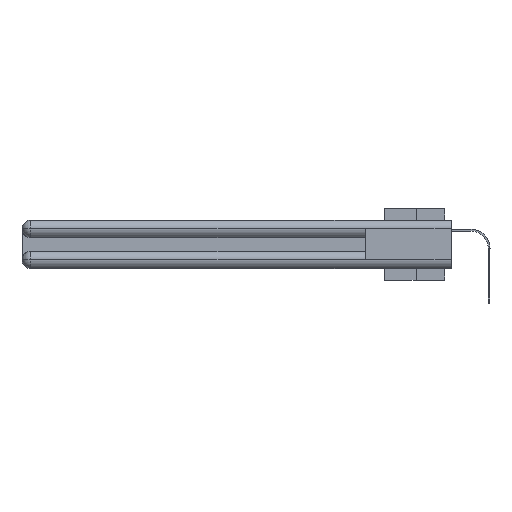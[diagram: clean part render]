
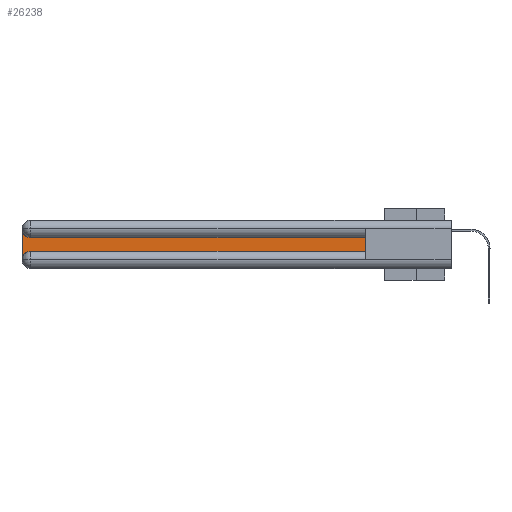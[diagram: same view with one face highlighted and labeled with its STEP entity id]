
A CAD part, left-side view. The second image highlights one B-rep face of the part: STEP entity #26238.
In plain terms, the highlighted planar face has unit normal (-1, 0, 0).
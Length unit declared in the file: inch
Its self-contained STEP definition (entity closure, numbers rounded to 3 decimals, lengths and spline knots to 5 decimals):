
#18 = CARTESIAN_POINT ( 'NONE',  ( 0.075, 2.94, -0.2775 ) ) ;
#342 = CIRCLE ( 'NONE', #5447, 0.06 ) ;
#403 = ORIENTED_EDGE ( 'NONE', *, *, #12688, .T. ) ;
#964 = CARTESIAN_POINT ( 'NONE',  ( 0.075, 0.6, -0.2175 ) ) ;
#1735 = LINE ( 'NONE', #29291, #29324 ) ;
#1938 = VERTEX_POINT ( 'NONE', #13409 ) ;
#2490 = VERTEX_POINT ( 'NONE', #15126 ) ;
#3595 = VERTEX_POINT ( 'NONE', #4472 ) ;
#3996 = DIRECTION ( 'NONE',  ( 0., -1., 0. ) ) ;
#4472 = CARTESIAN_POINT ( 'NONE',  ( 0.075, 3., -0.2775 ) ) ;
#5447 = AXIS2_PLACEMENT_3D ( 'NONE', #18, #12202, #24396 ) ;
#5637 = ORIENTED_EDGE ( 'NONE', *, *, #17181, .T. ) ;
#7115 = EDGE_CURVE ( 'NONE', #2490, #18605, #31381, .T. ) ;
#8290 = VERTEX_POINT ( 'NONE', #36392 ) ;
#10397 = CARTESIAN_POINT ( 'NONE',  ( 0.075, 0.6, -0.1225 ) ) ;
#10613 = DIRECTION ( 'NONE',  ( 0., 1., 0. ) ) ;
#11081 = EDGE_LOOP ( 'NONE', ( #22307, #5637, #36394, #403, #11160, #30911 ) ) ;
#11160 = ORIENTED_EDGE ( 'NONE', *, *, #7115, .T. ) ;
#12202 = DIRECTION ( 'NONE',  ( 1., 0., 0. ) ) ;
#12688 = EDGE_CURVE ( 'NONE', #3595, #2490, #342, .T. ) ;
#13157 = DIRECTION ( 'NONE',  ( 0., 0., -1. ) ) ;
#13409 = CARTESIAN_POINT ( 'NONE',  ( 0.075, 2.94, -0.1225 ) ) ;
#13956 = EDGE_CURVE ( 'NONE', #14171, #1938, #31977, .T. ) ;
#14117 = FACE_OUTER_BOUND ( 'NONE', #11081, .T. ) ;
#14171 = VERTEX_POINT ( 'NONE', #35559 ) ;
#15126 = CARTESIAN_POINT ( 'NONE',  ( 0.075, 2.94, -0.2175 ) ) ;
#15344 = AXIS2_PLACEMENT_3D ( 'NONE', #32674, #19718, #37900 ) ;
#15754 = VECTOR ( 'NONE', #10613, 39.37008 ) ;
#17181 = EDGE_CURVE ( 'NONE', #1938, #8290, #27856, .T. ) ;
#18309 = EDGE_CURVE ( 'NONE', #18605, #14171, #26946, .T. ) ;
#18605 = VERTEX_POINT ( 'NONE', #964 ) ;
#19331 = CARTESIAN_POINT ( 'NONE',  ( 0.075, 2.94, -0.0625 ) ) ;
#19718 = DIRECTION ( 'NONE',  ( 1., 0., 0. ) ) ;
#20832 = AXIS2_PLACEMENT_3D ( 'NONE', #19331, #22746, #13157 ) ;
#22307 = ORIENTED_EDGE ( 'NONE', *, *, #13956, .T. ) ;
#22746 = DIRECTION ( 'NONE',  ( 1., 0., 0. ) ) ;
#23088 = DIRECTION ( 'NONE',  ( 0., 0., -1. ) ) ;
#24396 = DIRECTION ( 'NONE',  ( 0., 0., -1. ) ) ;
#24948 = EDGE_CURVE ( 'NONE', #8290, #3595, #1735, .T. ) ;
#26238 = ADVANCED_FACE ( 'NONE', ( #14117 ), #38479, .F. ) ;
#26946 = LINE ( 'NONE', #39138, #27607 ) ;
#27607 = VECTOR ( 'NONE', #38549, 39.37008 ) ;
#27856 = CIRCLE ( 'NONE', #20832, 0.06 ) ;
#29291 = CARTESIAN_POINT ( 'NONE',  ( 0.075, 3., -0.2175 ) ) ;
#29324 = VECTOR ( 'NONE', #23088, 39.37008 ) ;
#30911 = ORIENTED_EDGE ( 'NONE', *, *, #18309, .T. ) ;
#31373 = VECTOR ( 'NONE', #3996, 39.37008 ) ;
#31381 = LINE ( 'NONE', #37566, #31373 ) ;
#31977 = LINE ( 'NONE', #10397, #15754 ) ;
#32674 = CARTESIAN_POINT ( 'NONE',  ( 0.075, 3., -0.1225 ) ) ;
#35559 = CARTESIAN_POINT ( 'NONE',  ( 0.075, 0.6, -0.1225 ) ) ;
#36392 = CARTESIAN_POINT ( 'NONE',  ( 0.075, 3., -0.0625 ) ) ;
#36394 = ORIENTED_EDGE ( 'NONE', *, *, #24948, .T. ) ;
#37566 = CARTESIAN_POINT ( 'NONE',  ( 0.075, 0.6, -0.2175 ) ) ;
#37900 = DIRECTION ( 'NONE',  ( 0., 0., -1. ) ) ;
#38479 = PLANE ( 'NONE',  #15344 ) ;
#38549 = DIRECTION ( 'NONE',  ( 0., 0., 1. ) ) ;
#39138 = CARTESIAN_POINT ( 'NONE',  ( 0.075, 0.6, -0.2175 ) ) ;
